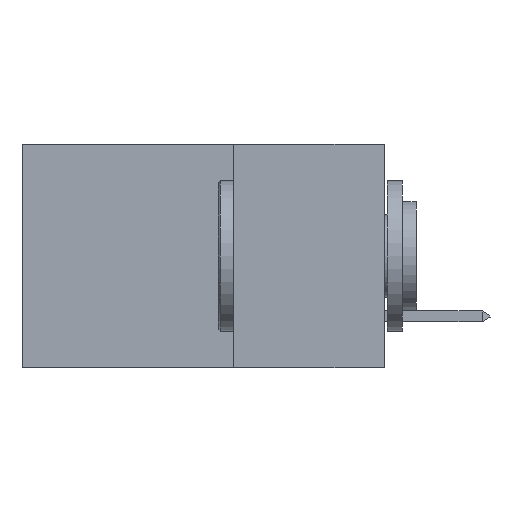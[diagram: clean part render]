
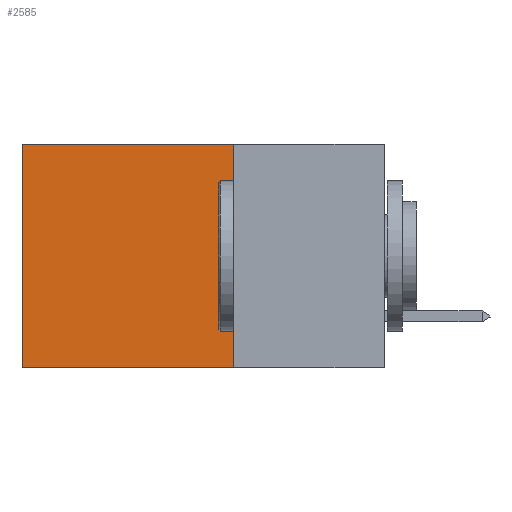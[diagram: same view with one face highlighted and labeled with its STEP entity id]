
A CAD part, left-side view. The second image highlights one B-rep face of the part: STEP entity #2585.
In plain terms, the highlighted planar face has unit normal (-1, 0, 0).
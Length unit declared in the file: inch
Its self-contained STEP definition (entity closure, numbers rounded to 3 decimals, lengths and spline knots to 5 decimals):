
#1065 = CARTESIAN_POINT ( 'NONE',  ( 0.2875, 0.6, 0. ) ) ;
#1996 = LINE ( 'NONE', #22507, #10245 ) ;
#2065 = CARTESIAN_POINT ( 'NONE',  ( 0.2875, 0.25, -0.37 ) ) ;
#2585 = ADVANCED_FACE ( 'NONE', ( #13391 ), #27903, .F. ) ;
#4087 = VECTOR ( 'NONE', #34866, 39.37008 ) ;
#4123 = EDGE_CURVE ( 'NONE', #8532, #12049, #6286, .T. ) ;
#5053 = CARTESIAN_POINT ( 'NONE',  ( 0.2875, 0.25, 0. ) ) ;
#5131 = DIRECTION ( 'NONE',  ( 0., 0., -1. ) ) ;
#5742 = EDGE_LOOP ( 'NONE', ( #35691, #11411, #18516, #23069 ) ) ;
#6286 = LINE ( 'NONE', #1065, #4087 ) ;
#8532 = VERTEX_POINT ( 'NONE', #12486 ) ;
#10245 = VECTOR ( 'NONE', #25797, 39.37008 ) ;
#11300 = LINE ( 'NONE', #26951, #17388 ) ;
#11411 = ORIENTED_EDGE ( 'NONE', *, *, #24732, .F. ) ;
#11695 = AXIS2_PLACEMENT_3D ( 'NONE', #28130, #30680, #16862 ) ;
#12049 = VERTEX_POINT ( 'NONE', #31489 ) ;
#12170 = CARTESIAN_POINT ( 'NONE',  ( 0.2875, 0.25, 0. ) ) ;
#12289 = DIRECTION ( 'NONE',  ( 0., 1., 0. ) ) ;
#12486 = CARTESIAN_POINT ( 'NONE',  ( 0.2875, 0.6, 0. ) ) ;
#13391 = FACE_OUTER_BOUND ( 'NONE', #5742, .T. ) ;
#15456 = VERTEX_POINT ( 'NONE', #5053 ) ;
#16862 = DIRECTION ( 'NONE',  ( 0., 0., -1. ) ) ;
#17109 = LINE ( 'NONE', #12170, #20599 ) ;
#17388 = VECTOR ( 'NONE', #5131, 39.37008 ) ;
#18516 = ORIENTED_EDGE ( 'NONE', *, *, #25459, .F. ) ;
#20599 = VECTOR ( 'NONE', #12289, 39.37008 ) ;
#22507 = CARTESIAN_POINT ( 'NONE',  ( 0.2875, 0.25, -0.37 ) ) ;
#23069 = ORIENTED_EDGE ( 'NONE', *, *, #29620, .T. ) ;
#24732 = EDGE_CURVE ( 'NONE', #29824, #12049, #1996, .T. ) ;
#25459 = EDGE_CURVE ( 'NONE', #15456, #29824, #11300, .T. ) ;
#25797 = DIRECTION ( 'NONE',  ( 0., 1., 0. ) ) ;
#26951 = CARTESIAN_POINT ( 'NONE',  ( 0.2875, 0.25, 0. ) ) ;
#27903 = PLANE ( 'NONE',  #11695 ) ;
#28130 = CARTESIAN_POINT ( 'NONE',  ( 0.2875, 0.25, 0. ) ) ;
#29620 = EDGE_CURVE ( 'NONE', #15456, #8532, #17109, .T. ) ;
#29824 = VERTEX_POINT ( 'NONE', #2065 ) ;
#30680 = DIRECTION ( 'NONE',  ( 1., 0., 0. ) ) ;
#31489 = CARTESIAN_POINT ( 'NONE',  ( 0.2875, 0.6, -0.37 ) ) ;
#34866 = DIRECTION ( 'NONE',  ( 0., 0., -1. ) ) ;
#35691 = ORIENTED_EDGE ( 'NONE', *, *, #4123, .T. ) ;
